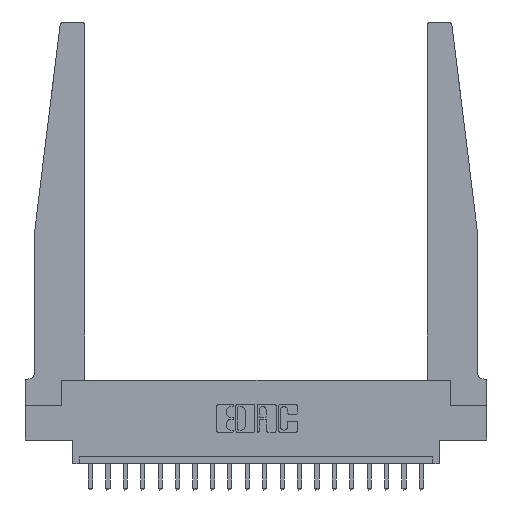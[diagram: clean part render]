
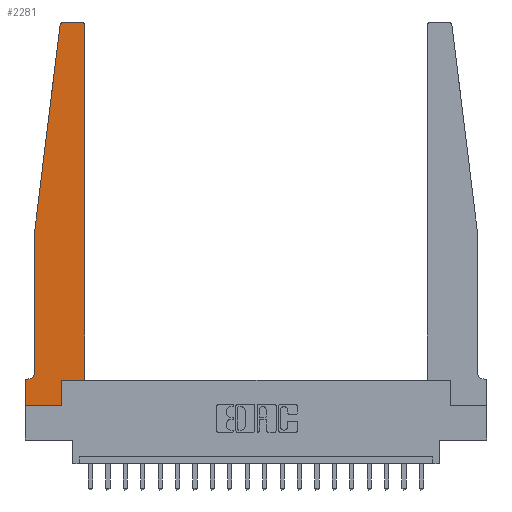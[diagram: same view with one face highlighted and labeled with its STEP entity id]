
A CAD part, top view. The second image highlights one B-rep face of the part: STEP entity #2281.
In plain terms, the highlighted planar face has unit normal (0, 0, 1).
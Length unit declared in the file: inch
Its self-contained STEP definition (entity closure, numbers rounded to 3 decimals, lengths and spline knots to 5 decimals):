
#374 = VERTEX_POINT ( 'NONE', #9832 ) ;
#596 = ORIENTED_EDGE ( 'NONE', *, *, #18638, .T. ) ;
#896 = EDGE_CURVE ( 'NONE', #1423, #16957, #18810, .T. ) ;
#975 = VECTOR ( 'NONE', #17145, 39.37008 ) ;
#1257 = VERTEX_POINT ( 'NONE', #19274 ) ;
#1277 = CIRCLE ( 'NONE', #15241, 0.03 ) ;
#1423 = VERTEX_POINT ( 'NONE', #7890 ) ;
#1550 = DIRECTION ( 'NONE',  ( 0., 0., 1. ) ) ;
#1700 = LINE ( 'NONE', #5512, #9067 ) ;
#1817 = DIRECTION ( 'NONE',  ( 1., 0., 0. ) ) ;
#2270 = CARTESIAN_POINT ( 'NONE',  ( 0.065, 0.1875, 0.37 ) ) ;
#2281 = ADVANCED_FACE ( 'NONE', ( #5217 ), #6871, .T. ) ;
#2374 = CARTESIAN_POINT ( 'NONE',  ( 0.425, 0.18, 0.37 ) ) ;
#2612 = CARTESIAN_POINT ( 'NONE',  ( 0.015, 0.1875, 0.37 ) ) ;
#2740 = LINE ( 'NONE', #18389, #11613 ) ;
#2746 = AXIS2_PLACEMENT_3D ( 'NONE', #13180, #14888, #5233 ) ;
#3821 = LINE ( 'NONE', #17484, #6473 ) ;
#3863 = DIRECTION ( 'NONE',  ( -1., 0., 0. ) ) ;
#4136 = LINE ( 'NONE', #11058, #16180 ) ;
#4686 = EDGE_CURVE ( 'NONE', #6809, #17662, #11823, .T. ) ;
#5211 = CARTESIAN_POINT ( 'NONE',  ( 0.425, 2.72, 0.37 ) ) ;
#5217 = FACE_OUTER_BOUND ( 'NONE', #10293, .T. ) ;
#5233 = DIRECTION ( 'NONE',  ( 1., 0., 0. ) ) ;
#5396 = VECTOR ( 'NONE', #7148, 39.37008 ) ;
#5512 = CARTESIAN_POINT ( 'NONE',  ( 0., 0., 0.37 ) ) ;
#5518 = CARTESIAN_POINT ( 'NONE',  ( 0.425, 0.18, 0.37 ) ) ;
#6255 = CIRCLE ( 'NONE', #20260, 0.05 ) ;
#6382 = DIRECTION ( 'NONE',  ( 0., 0., -1. ) ) ;
#6473 = VECTOR ( 'NONE', #19007, 39.37008 ) ;
#6809 = VERTEX_POINT ( 'NONE', #2612 ) ;
#6871 = PLANE ( 'NONE',  #2746 ) ;
#7136 = CARTESIAN_POINT ( 'NONE',  ( 0.2605, 0.18, 0.37 ) ) ;
#7148 = DIRECTION ( 'NONE',  ( 1., 0., 0. ) ) ;
#7561 = EDGE_CURVE ( 'NONE', #11163, #13151, #12186, .T. ) ;
#7861 = DIRECTION ( 'NONE',  ( -1., 0., 0. ) ) ;
#7890 = CARTESIAN_POINT ( 'NONE',  ( 0.24675, 2.72367, 0.37 ) ) ;
#7947 = DIRECTION ( 'NONE',  ( 0., -1., 0. ) ) ;
#8353 = ORIENTED_EDGE ( 'NONE', *, *, #19602, .T. ) ;
#9067 = VECTOR ( 'NONE', #18045, 39.37008 ) ;
#9179 = ORIENTED_EDGE ( 'NONE', *, *, #15455, .T. ) ;
#9319 = LINE ( 'NONE', #19146, #975 ) ;
#9364 = DIRECTION ( 'NONE',  ( 0., 1., 0. ) ) ;
#9564 = CARTESIAN_POINT ( 'NONE',  ( 0.27653, 2.75, 0.37 ) ) ;
#9637 = CARTESIAN_POINT ( 'NONE',  ( 0.015, 0.2375, 0.37 ) ) ;
#9832 = CARTESIAN_POINT ( 'NONE',  ( 0., 0., 0.37 ) ) ;
#9878 = EDGE_CURVE ( 'NONE', #17890, #11163, #1277, .T. ) ;
#10205 = VECTOR ( 'NONE', #18740, 39.37008 ) ;
#10293 = EDGE_LOOP ( 'NONE', ( #11244, #9179, #10425, #8353, #14273, #16202, #15712, #596, #19222, #15215, #18244, #16032 ) ) ;
#10425 = ORIENTED_EDGE ( 'NONE', *, *, #896, .T. ) ;
#10706 = AXIS2_PLACEMENT_3D ( 'NONE', #10960, #1550, #12557 ) ;
#10960 = CARTESIAN_POINT ( 'NONE',  ( 0.27653, 2.72, 0.37 ) ) ;
#11058 = CARTESIAN_POINT ( 'NONE',  ( 0.065, 1.25, 0.37 ) ) ;
#11163 = VERTEX_POINT ( 'NONE', #15993 ) ;
#11244 = ORIENTED_EDGE ( 'NONE', *, *, #7561, .T. ) ;
#11277 = VERTEX_POINT ( 'NONE', #17706 ) ;
#11613 = VECTOR ( 'NONE', #9364, 39.37008 ) ;
#11823 = LINE ( 'NONE', #2270, #18207 ) ;
#12040 = VERTEX_POINT ( 'NONE', #7136 ) ;
#12186 = LINE ( 'NONE', #18871, #10205 ) ;
#12557 = DIRECTION ( 'NONE',  ( 1., 0., 0. ) ) ;
#12997 = CIRCLE ( 'NONE', #10706, 0.03 ) ;
#13151 = VERTEX_POINT ( 'NONE', #9564 ) ;
#13180 = CARTESIAN_POINT ( 'NONE',  ( 0., 0.1875, 0.37 ) ) ;
#14057 = CARTESIAN_POINT ( 'NONE',  ( 0., 0.1875, 0.37 ) ) ;
#14273 = ORIENTED_EDGE ( 'NONE', *, *, #20141, .T. ) ;
#14415 = DIRECTION ( 'NONE',  ( 0., 0., 1. ) ) ;
#14419 = VECTOR ( 'NONE', #20264, 39.37008 ) ;
#14856 = EDGE_CURVE ( 'NONE', #17662, #374, #3821, .T. ) ;
#14888 = DIRECTION ( 'NONE',  ( 0., 0., 1. ) ) ;
#15215 = ORIENTED_EDGE ( 'NONE', *, *, #18608, .T. ) ;
#15241 = AXIS2_PLACEMENT_3D ( 'NONE', #19136, #14415, #1817 ) ;
#15455 = EDGE_CURVE ( 'NONE', #13151, #1423, #12997, .T. ) ;
#15515 = CARTESIAN_POINT ( 'NONE',  ( 0.065, 1.25, 0.37 ) ) ;
#15712 = ORIENTED_EDGE ( 'NONE', *, *, #14856, .T. ) ;
#15993 = CARTESIAN_POINT ( 'NONE',  ( 0.395, 2.75, 0.37 ) ) ;
#16032 = ORIENTED_EDGE ( 'NONE', *, *, #9878, .T. ) ;
#16180 = VECTOR ( 'NONE', #7947, 39.37008 ) ;
#16202 = ORIENTED_EDGE ( 'NONE', *, *, #4686, .T. ) ;
#16957 = VERTEX_POINT ( 'NONE', #15515 ) ;
#17034 = EDGE_CURVE ( 'NONE', #18928, #17890, #2740, .T. ) ;
#17145 = DIRECTION ( 'NONE',  ( 0., 1., 0. ) ) ;
#17484 = CARTESIAN_POINT ( 'NONE',  ( 0., 0., 0.37 ) ) ;
#17662 = VERTEX_POINT ( 'NONE', #14057 ) ;
#17706 = CARTESIAN_POINT ( 'NONE',  ( 0.065, 0.2375, 0.37 ) ) ;
#17890 = VERTEX_POINT ( 'NONE', #5211 ) ;
#18045 = DIRECTION ( 'NONE',  ( 1., 0., 0. ) ) ;
#18207 = VECTOR ( 'NONE', #3863, 39.37008 ) ;
#18244 = ORIENTED_EDGE ( 'NONE', *, *, #17034, .T. ) ;
#18389 = CARTESIAN_POINT ( 'NONE',  ( 0.425, 0.18, 0.37 ) ) ;
#18420 = EDGE_CURVE ( 'NONE', #1257, #12040, #9319, .T. ) ;
#18608 = EDGE_CURVE ( 'NONE', #12040, #18928, #19421, .T. ) ;
#18623 = CARTESIAN_POINT ( 'NONE',  ( 0.065, 1.25, 0.37 ) ) ;
#18638 = EDGE_CURVE ( 'NONE', #374, #1257, #1700, .T. ) ;
#18740 = DIRECTION ( 'NONE',  ( -1., 0., 0. ) ) ;
#18810 = LINE ( 'NONE', #18623, #14419 ) ;
#18871 = CARTESIAN_POINT ( 'NONE',  ( 0.25, 2.75, 0.37 ) ) ;
#18928 = VERTEX_POINT ( 'NONE', #5518 ) ;
#19007 = DIRECTION ( 'NONE',  ( 0., -1., 0. ) ) ;
#19136 = CARTESIAN_POINT ( 'NONE',  ( 0.395, 2.72, 0.37 ) ) ;
#19146 = CARTESIAN_POINT ( 'NONE',  ( 0.2605, 0.18, 0.37 ) ) ;
#19222 = ORIENTED_EDGE ( 'NONE', *, *, #18420, .T. ) ;
#19274 = CARTESIAN_POINT ( 'NONE',  ( 0.2605, 0., 0.37 ) ) ;
#19421 = LINE ( 'NONE', #2374, #5396 ) ;
#19602 = EDGE_CURVE ( 'NONE', #16957, #11277, #4136, .T. ) ;
#20141 = EDGE_CURVE ( 'NONE', #11277, #6809, #6255, .T. ) ;
#20260 = AXIS2_PLACEMENT_3D ( 'NONE', #9637, #6382, #7861 ) ;
#20264 = DIRECTION ( 'NONE',  ( -0.122, -0.992, 0. ) ) ;
